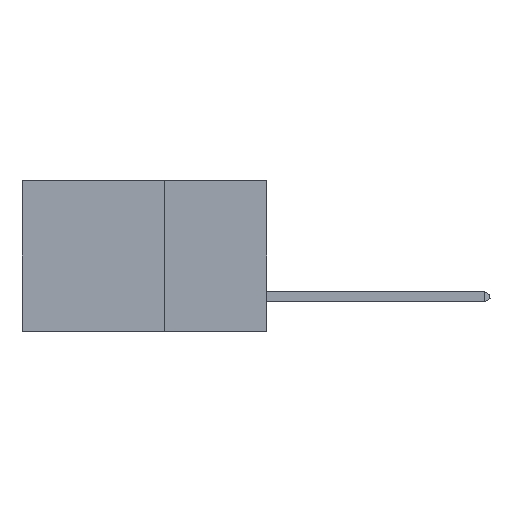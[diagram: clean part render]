
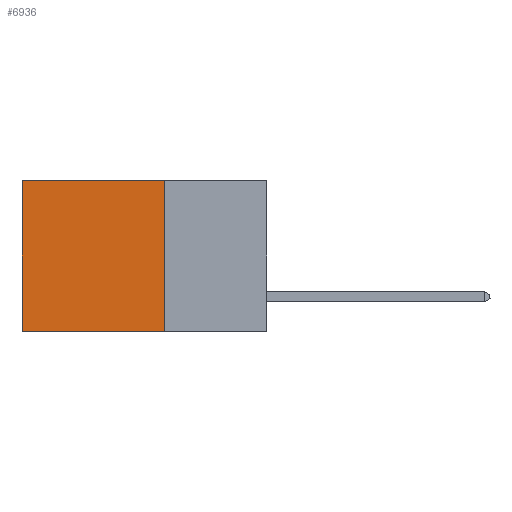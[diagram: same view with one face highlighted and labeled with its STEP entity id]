
A CAD part, left-side view. The second image highlights one B-rep face of the part: STEP entity #6936.
In plain terms, the highlighted planar face has unit normal (-1, 0, 0).
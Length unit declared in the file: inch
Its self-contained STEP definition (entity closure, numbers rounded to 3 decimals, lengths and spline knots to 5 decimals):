
#77 = VERTEX_POINT ( 'NONE', #16503 ) ;
#3614 = LINE ( 'NONE', #12275, #22022 ) ;
#4063 = ORIENTED_EDGE ( 'NONE', *, *, #13504, .F. ) ;
#6936 = ADVANCED_FACE ( 'NONE', ( #25788 ), #35826, .F. ) ;
#9098 = VECTOR ( 'NONE', #25236, 39.37008 ) ;
#9375 = EDGE_CURVE ( 'NONE', #16547, #17965, #22458, .T. ) ;
#9449 = DIRECTION ( 'NONE',  ( 0., 1., 0. ) ) ;
#12275 = CARTESIAN_POINT ( 'NONE',  ( 0.2875, 0.25, 0. ) ) ;
#12636 = CARTESIAN_POINT ( 'NONE',  ( 0.2875, 0.6, 0. ) ) ;
#12652 = CARTESIAN_POINT ( 'NONE',  ( 0.2875, 0.25, 0. ) ) ;
#13504 = EDGE_CURVE ( 'NONE', #17965, #13703, #33695, .T. ) ;
#13703 = VERTEX_POINT ( 'NONE', #35452 ) ;
#13887 = EDGE_CURVE ( 'NONE', #16547, #77, #3614, .T. ) ;
#14742 = VECTOR ( 'NONE', #28161, 39.37008 ) ;
#14975 = DIRECTION ( 'NONE',  ( 0., 1., 0. ) ) ;
#15718 = ORIENTED_EDGE ( 'NONE', *, *, #9375, .F. ) ;
#16093 = ORIENTED_EDGE ( 'NONE', *, *, #13887, .T. ) ;
#16503 = CARTESIAN_POINT ( 'NONE',  ( 0.2875, 0.6, 0. ) ) ;
#16538 = DIRECTION ( 'NONE',  ( 0., 0., -1. ) ) ;
#16547 = VERTEX_POINT ( 'NONE', #12652 ) ;
#17647 = CARTESIAN_POINT ( 'NONE',  ( 0.2875, 0.25, -0.37 ) ) ;
#17965 = VERTEX_POINT ( 'NONE', #17647 ) ;
#18375 = EDGE_CURVE ( 'NONE', #77, #13703, #23413, .T. ) ;
#22022 = VECTOR ( 'NONE', #9449, 39.37008 ) ;
#22458 = LINE ( 'NONE', #36528, #14742 ) ;
#23413 = LINE ( 'NONE', #12636, #9098 ) ;
#25236 = DIRECTION ( 'NONE',  ( 0., 0., -1. ) ) ;
#25788 = FACE_OUTER_BOUND ( 'NONE', #35339, .T. ) ;
#28161 = DIRECTION ( 'NONE',  ( 0., 0., -1. ) ) ;
#31627 = AXIS2_PLACEMENT_3D ( 'NONE', #36865, #32628, #16538 ) ;
#31787 = CARTESIAN_POINT ( 'NONE',  ( 0.2875, 0.25, -0.37 ) ) ;
#32628 = DIRECTION ( 'NONE',  ( 1., 0., 0. ) ) ;
#32754 = VECTOR ( 'NONE', #14975, 39.37008 ) ;
#33695 = LINE ( 'NONE', #31787, #32754 ) ;
#35339 = EDGE_LOOP ( 'NONE', ( #35707, #4063, #15718, #16093 ) ) ;
#35452 = CARTESIAN_POINT ( 'NONE',  ( 0.2875, 0.6, -0.37 ) ) ;
#35707 = ORIENTED_EDGE ( 'NONE', *, *, #18375, .T. ) ;
#35826 = PLANE ( 'NONE',  #31627 ) ;
#36528 = CARTESIAN_POINT ( 'NONE',  ( 0.2875, 0.25, 0. ) ) ;
#36865 = CARTESIAN_POINT ( 'NONE',  ( 0.2875, 0.25, 0. ) ) ;
